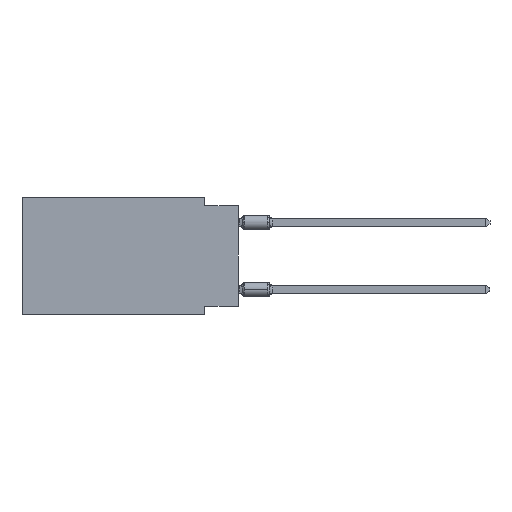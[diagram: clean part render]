
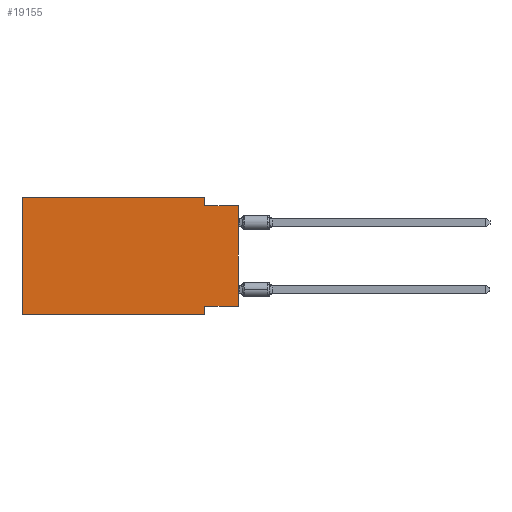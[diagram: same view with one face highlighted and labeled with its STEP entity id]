
A CAD part, left-side view. The second image highlights one B-rep face of the part: STEP entity #19155.
In plain terms, the highlighted planar face has unit normal (-1, 0, 0).
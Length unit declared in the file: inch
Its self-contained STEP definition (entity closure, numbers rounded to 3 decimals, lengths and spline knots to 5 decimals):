
#52 = ORIENTED_EDGE ( 'NONE', *, *, #9478, .F. ) ;
#658 = LINE ( 'NONE', #25492, #27496 ) ;
#710 = LINE ( 'NONE', #25692, #14779 ) ;
#859 = DIRECTION ( 'NONE',  ( 0., 0., 1. ) ) ;
#1483 = LINE ( 'NONE', #1627, #26161 ) ;
#1627 = CARTESIAN_POINT ( 'NONE',  ( 0., 0.645, -0.35 ) ) ;
#1735 = DIRECTION ( 'NONE',  ( 0., 0., 1. ) ) ;
#2397 = CARTESIAN_POINT ( 'NONE',  ( 0., 0.1, 0. ) ) ;
#4005 = ORIENTED_EDGE ( 'NONE', *, *, #13086, .F. ) ;
#4560 = CARTESIAN_POINT ( 'NONE',  ( 0., 0.1, -0.325 ) ) ;
#4603 = CARTESIAN_POINT ( 'NONE',  ( 0., 0., -0.025 ) ) ;
#4972 = DIRECTION ( 'NONE',  ( 0., -1., 0. ) ) ;
#6138 = EDGE_LOOP ( 'NONE', ( #28526, #19006, #52, #25557, #10552, #25225, #7528, #4005 ) ) ;
#6432 = VERTEX_POINT ( 'NONE', #4560 ) ;
#6647 = LINE ( 'NONE', #22530, #11938 ) ;
#7528 = ORIENTED_EDGE ( 'NONE', *, *, #21646, .F. ) ;
#8719 = CARTESIAN_POINT ( 'NONE',  ( 0., 0.645, 0. ) ) ;
#9400 = FACE_OUTER_BOUND ( 'NONE', #6138, .T. ) ;
#9478 = EDGE_CURVE ( 'NONE', #15473, #16379, #11064, .T. ) ;
#9553 = DIRECTION ( 'NONE',  ( 1., 0., 0. ) ) ;
#9992 = CARTESIAN_POINT ( 'NONE',  ( 0., 0.645, 0. ) ) ;
#10386 = VECTOR ( 'NONE', #12175, 39.37008 ) ;
#10552 = ORIENTED_EDGE ( 'NONE', *, *, #14569, .F. ) ;
#11064 = LINE ( 'NONE', #15515, #11222 ) ;
#11170 = DIRECTION ( 'NONE',  ( 0., -1., 0. ) ) ;
#11222 = VECTOR ( 'NONE', #15221, 39.37008 ) ;
#11380 = EDGE_CURVE ( 'NONE', #16379, #25386, #14119, .T. ) ;
#11643 = DIRECTION ( 'NONE',  ( 0., 0., -1. ) ) ;
#11938 = VECTOR ( 'NONE', #1735, 39.37008 ) ;
#12175 = DIRECTION ( 'NONE',  ( 0., 0., -1. ) ) ;
#13086 = EDGE_CURVE ( 'NONE', #20966, #6432, #13439, .T. ) ;
#13174 = PLANE ( 'NONE',  #18840 ) ;
#13439 = LINE ( 'NONE', #22485, #19992 ) ;
#14119 = LINE ( 'NONE', #4603, #26532 ) ;
#14569 = EDGE_CURVE ( 'NONE', #22938, #20178, #6647, .T. ) ;
#14577 = CARTESIAN_POINT ( 'NONE',  ( 0., 0., -0.025 ) ) ;
#14779 = VECTOR ( 'NONE', #859, 39.37008 ) ;
#14990 = CARTESIAN_POINT ( 'NONE',  ( 0., 0.645, -0.35 ) ) ;
#15221 = DIRECTION ( 'NONE',  ( 0., 0., -1. ) ) ;
#15473 = VERTEX_POINT ( 'NONE', #2397 ) ;
#15515 = CARTESIAN_POINT ( 'NONE',  ( 0., 0.1, 0. ) ) ;
#15724 = EDGE_CURVE ( 'NONE', #22938, #25869, #1483, .T. ) ;
#15900 = EDGE_CURVE ( 'NONE', #20966, #25386, #710, .T. ) ;
#15956 = CARTESIAN_POINT ( 'NONE',  ( 0., 0., -0.325 ) ) ;
#15975 = DIRECTION ( 'NONE',  ( 0., 1., 0. ) ) ;
#16379 = VERTEX_POINT ( 'NONE', #21615 ) ;
#18723 = CARTESIAN_POINT ( 'NONE',  ( 0., 0.1, -0.35 ) ) ;
#18840 = AXIS2_PLACEMENT_3D ( 'NONE', #8719, #9553, #11643 ) ;
#19006 = ORIENTED_EDGE ( 'NONE', *, *, #11380, .F. ) ;
#19155 = ADVANCED_FACE ( 'NONE', ( #9400 ), #13174, .F. ) ;
#19472 = CARTESIAN_POINT ( 'NONE',  ( 0., 0.1, -0.35 ) ) ;
#19992 = VECTOR ( 'NONE', #15975, 39.37008 ) ;
#20178 = VERTEX_POINT ( 'NONE', #9992 ) ;
#20966 = VERTEX_POINT ( 'NONE', #15956 ) ;
#21615 = CARTESIAN_POINT ( 'NONE',  ( 0., 0.1, -0.025 ) ) ;
#21646 = EDGE_CURVE ( 'NONE', #6432, #25869, #28205, .T. ) ;
#22485 = CARTESIAN_POINT ( 'NONE',  ( 0., 0., -0.325 ) ) ;
#22530 = CARTESIAN_POINT ( 'NONE',  ( 0., 0.645, 0. ) ) ;
#22938 = VERTEX_POINT ( 'NONE', #14990 ) ;
#23183 = EDGE_CURVE ( 'NONE', #20178, #15473, #658, .T. ) ;
#25225 = ORIENTED_EDGE ( 'NONE', *, *, #15724, .T. ) ;
#25386 = VERTEX_POINT ( 'NONE', #14577 ) ;
#25492 = CARTESIAN_POINT ( 'NONE',  ( 0., 0.645, 0. ) ) ;
#25557 = ORIENTED_EDGE ( 'NONE', *, *, #23183, .F. ) ;
#25692 = CARTESIAN_POINT ( 'NONE',  ( 0., 0., 0. ) ) ;
#25869 = VERTEX_POINT ( 'NONE', #18723 ) ;
#26161 = VECTOR ( 'NONE', #11170, 39.37008 ) ;
#26532 = VECTOR ( 'NONE', #27361, 39.37008 ) ;
#27361 = DIRECTION ( 'NONE',  ( 0., -1., 0. ) ) ;
#27496 = VECTOR ( 'NONE', #4972, 39.37008 ) ;
#28205 = LINE ( 'NONE', #19472, #10386 ) ;
#28526 = ORIENTED_EDGE ( 'NONE', *, *, #15900, .T. ) ;
